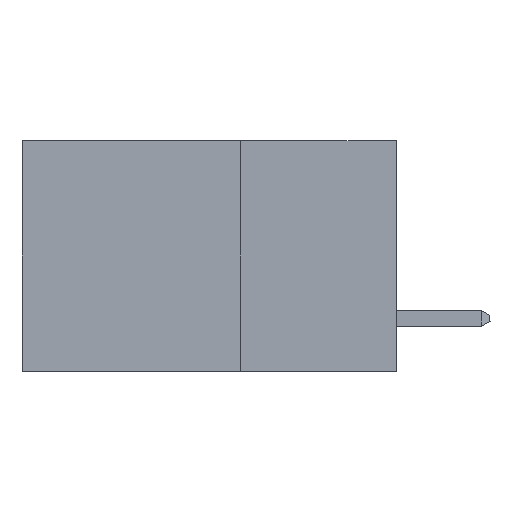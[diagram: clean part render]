
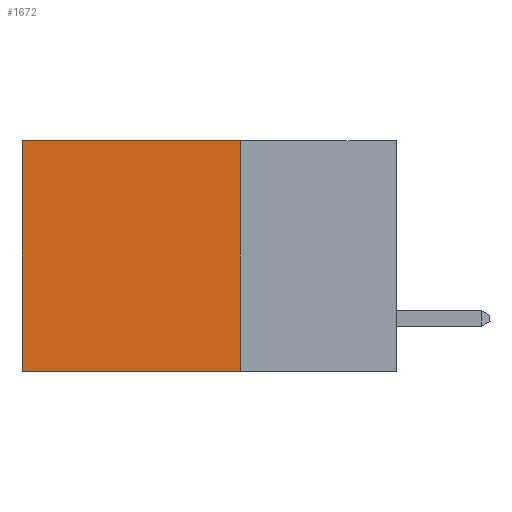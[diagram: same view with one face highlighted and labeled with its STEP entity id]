
A CAD part, left-side view. The second image highlights one B-rep face of the part: STEP entity #1672.
In plain terms, the highlighted planar face has unit normal (-1, 0, 0).
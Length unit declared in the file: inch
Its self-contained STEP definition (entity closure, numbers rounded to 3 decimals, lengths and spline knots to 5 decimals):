
#48 = EDGE_CURVE ( 'NONE', #10661, #12847, #7328, .T. ) ;
#296 = CARTESIAN_POINT ( 'NONE',  ( 0.298, 0.25, 0. ) ) ;
#830 = EDGE_CURVE ( 'NONE', #10661, #9811, #11551, .T. ) ;
#1485 = CARTESIAN_POINT ( 'NONE',  ( 0.298, 0.6, 0. ) ) ;
#1672 = ADVANCED_FACE ( 'NONE', ( #3066 ), #12476, .F. ) ;
#2086 = AXIS2_PLACEMENT_3D ( 'NONE', #13661, #6563, #7779 ) ;
#2723 = DIRECTION ( 'NONE',  ( 0., 1., 0. ) ) ;
#3066 = FACE_OUTER_BOUND ( 'NONE', #11109, .T. ) ;
#3619 = CARTESIAN_POINT ( 'NONE',  ( 0.298, 0.6, 0. ) ) ;
#3718 = CARTESIAN_POINT ( 'NONE',  ( 0.298, 0.6, -0.37 ) ) ;
#4399 = VERTEX_POINT ( 'NONE', #3718 ) ;
#5972 = DIRECTION ( 'NONE',  ( 0., 1., 0. ) ) ;
#6005 = ORIENTED_EDGE ( 'NONE', *, *, #830, .T. ) ;
#6563 = DIRECTION ( 'NONE',  ( 1., 0., 0. ) ) ;
#7328 = LINE ( 'NONE', #14937, #12510 ) ;
#7779 = DIRECTION ( 'NONE',  ( 0., 0., -1. ) ) ;
#7866 = DIRECTION ( 'NONE',  ( 0., 0., -1. ) ) ;
#9128 = VECTOR ( 'NONE', #5972, 39.37008 ) ;
#9530 = CARTESIAN_POINT ( 'NONE',  ( 0.298, 0.25, -0.37 ) ) ;
#9688 = DIRECTION ( 'NONE',  ( 0., 0., -1. ) ) ;
#9811 = VERTEX_POINT ( 'NONE', #3619 ) ;
#9997 = CARTESIAN_POINT ( 'NONE',  ( 0.298, 0.25, 0. ) ) ;
#10423 = EDGE_CURVE ( 'NONE', #9811, #4399, #15129, .T. ) ;
#10661 = VERTEX_POINT ( 'NONE', #9997 ) ;
#10818 = VECTOR ( 'NONE', #2723, 39.37008 ) ;
#11109 = EDGE_LOOP ( 'NONE', ( #13092, #11824, #13889, #6005 ) ) ;
#11218 = CARTESIAN_POINT ( 'NONE',  ( 0.298, 0.25, -0.37 ) ) ;
#11256 = VECTOR ( 'NONE', #9688, 39.37008 ) ;
#11551 = LINE ( 'NONE', #296, #10818 ) ;
#11824 = ORIENTED_EDGE ( 'NONE', *, *, #14145, .F. ) ;
#12476 = PLANE ( 'NONE',  #2086 ) ;
#12510 = VECTOR ( 'NONE', #7866, 39.37008 ) ;
#12847 = VERTEX_POINT ( 'NONE', #11218 ) ;
#13092 = ORIENTED_EDGE ( 'NONE', *, *, #10423, .T. ) ;
#13661 = CARTESIAN_POINT ( 'NONE',  ( 0.298, 0.25, 0. ) ) ;
#13889 = ORIENTED_EDGE ( 'NONE', *, *, #48, .F. ) ;
#14145 = EDGE_CURVE ( 'NONE', #12847, #4399, #14829, .T. ) ;
#14829 = LINE ( 'NONE', #9530, #9128 ) ;
#14937 = CARTESIAN_POINT ( 'NONE',  ( 0.298, 0.25, 0. ) ) ;
#15129 = LINE ( 'NONE', #1485, #11256 ) ;
